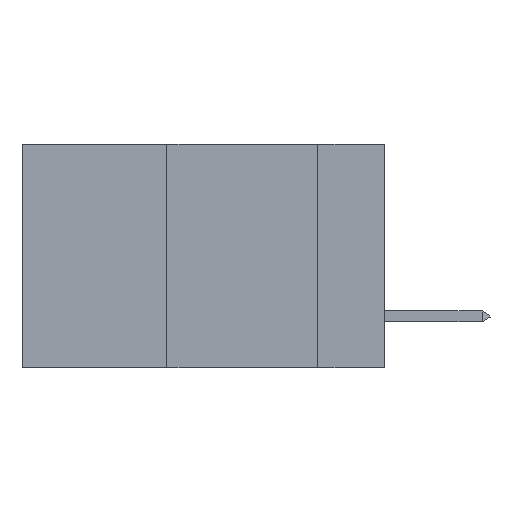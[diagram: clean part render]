
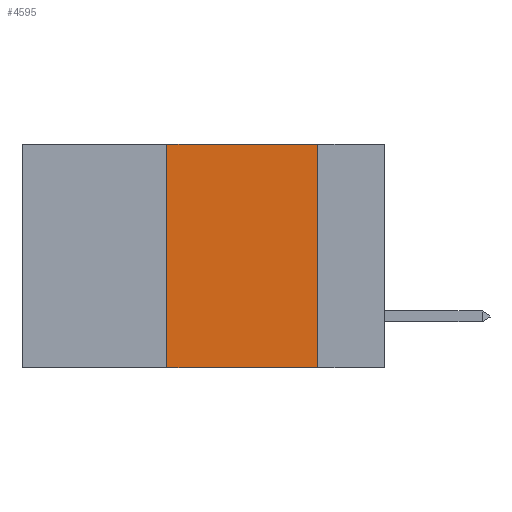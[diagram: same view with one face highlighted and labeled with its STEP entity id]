
A CAD part, left-side view. The second image highlights one B-rep face of the part: STEP entity #4595.
In plain terms, the highlighted planar face has unit normal (-1, 0, 0).
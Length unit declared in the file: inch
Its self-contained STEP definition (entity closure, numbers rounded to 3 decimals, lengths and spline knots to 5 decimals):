
#367 = CARTESIAN_POINT ( 'NONE',  ( 0., 0.6, -0.37 ) ) ;
#937 = PLANE ( 'NONE',  #25799 ) ;
#1237 = LINE ( 'NONE', #27914, #25014 ) ;
#1632 = VERTEX_POINT ( 'NONE', #18369 ) ;
#2204 = CARTESIAN_POINT ( 'NONE',  ( 0., 0.11, -0.37 ) ) ;
#3135 = DIRECTION ( 'NONE',  ( 0., 0., -1. ) ) ;
#4189 = CARTESIAN_POINT ( 'NONE',  ( 0., 0.11, 0. ) ) ;
#4595 = ADVANCED_FACE ( 'NONE', ( #25273 ), #937, .F. ) ;
#6838 = EDGE_CURVE ( 'NONE', #14486, #1632, #27381, .T. ) ;
#6972 = CARTESIAN_POINT ( 'NONE',  ( 0., 0.36, 0. ) ) ;
#7143 = LINE ( 'NONE', #367, #15644 ) ;
#8936 = DIRECTION ( 'NONE',  ( 0., -1., 0. ) ) ;
#9523 = EDGE_CURVE ( 'NONE', #14486, #27205, #7143, .T. ) ;
#10760 = VECTOR ( 'NONE', #19849, 39.37008 ) ;
#11487 = VERTEX_POINT ( 'NONE', #4189 ) ;
#13357 = ORIENTED_EDGE ( 'NONE', *, *, #9523, .T. ) ;
#13731 = VECTOR ( 'NONE', #8936, 39.37008 ) ;
#13744 = ORIENTED_EDGE ( 'NONE', *, *, #6838, .F. ) ;
#14486 = VERTEX_POINT ( 'NONE', #23747 ) ;
#14899 = DIRECTION ( 'NONE',  ( 0., 0., -1. ) ) ;
#15352 = CARTESIAN_POINT ( 'NONE',  ( 0., 0.6, 0. ) ) ;
#15644 = VECTOR ( 'NONE', #26454, 39.37008 ) ;
#16131 = CARTESIAN_POINT ( 'NONE',  ( 0., 0.6, 0. ) ) ;
#16471 = EDGE_CURVE ( 'NONE', #1632, #11487, #18462, .T. ) ;
#18369 = CARTESIAN_POINT ( 'NONE',  ( 0., 0.36, 0. ) ) ;
#18462 = LINE ( 'NONE', #15352, #13731 ) ;
#18648 = ORIENTED_EDGE ( 'NONE', *, *, #16471, .F. ) ;
#19849 = DIRECTION ( 'NONE',  ( 0., 0., 1. ) ) ;
#20442 = EDGE_CURVE ( 'NONE', #11487, #27205, #1237, .T. ) ;
#21723 = ORIENTED_EDGE ( 'NONE', *, *, #20442, .F. ) ;
#22570 = DIRECTION ( 'NONE',  ( 1., 0., 0. ) ) ;
#23747 = CARTESIAN_POINT ( 'NONE',  ( 0., 0.36, -0.37 ) ) ;
#24177 = EDGE_LOOP ( 'NONE', ( #21723, #18648, #13744, #13357 ) ) ;
#25014 = VECTOR ( 'NONE', #14899, 39.37008 ) ;
#25273 = FACE_OUTER_BOUND ( 'NONE', #24177, .T. ) ;
#25799 = AXIS2_PLACEMENT_3D ( 'NONE', #16131, #22570, #3135 ) ;
#26454 = DIRECTION ( 'NONE',  ( 0., -1., 0. ) ) ;
#27205 = VERTEX_POINT ( 'NONE', #2204 ) ;
#27381 = LINE ( 'NONE', #6972, #10760 ) ;
#27914 = CARTESIAN_POINT ( 'NONE',  ( 0., 0.11, 0. ) ) ;
